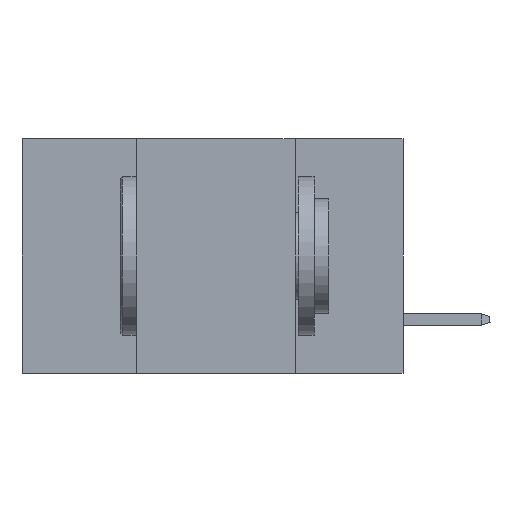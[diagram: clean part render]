
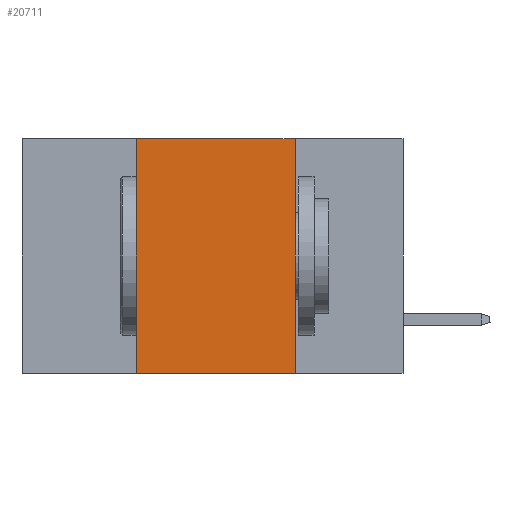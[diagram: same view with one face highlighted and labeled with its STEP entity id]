
A CAD part, left-side view. The second image highlights one B-rep face of the part: STEP entity #20711.
In plain terms, the highlighted planar face has unit normal (-1, 0, 0).
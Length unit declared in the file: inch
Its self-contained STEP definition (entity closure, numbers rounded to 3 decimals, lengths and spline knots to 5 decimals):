
#436 = EDGE_LOOP ( 'NONE', ( #23917, #10167, #9703, #27167 ) ) ;
#1954 = DIRECTION ( 'NONE',  ( 1., 0., 0. ) ) ;
#2016 = VECTOR ( 'NONE', #8291, 39.37008 ) ;
#4100 = VERTEX_POINT ( 'NONE', #9252 ) ;
#5850 = EDGE_CURVE ( 'NONE', #25699, #18921, #11287, .T. ) ;
#6035 = CARTESIAN_POINT ( 'NONE',  ( 0., 0.42, 0. ) ) ;
#6901 = EDGE_CURVE ( 'NONE', #18921, #4100, #20561, .T. ) ;
#7344 = DIRECTION ( 'NONE',  ( 0., -1., 0. ) ) ;
#7386 = DIRECTION ( 'NONE',  ( 0., -1., 0. ) ) ;
#8291 = DIRECTION ( 'NONE',  ( 0., 0., -1. ) ) ;
#9195 = CARTESIAN_POINT ( 'NONE',  ( 0., 0.6, -0.37 ) ) ;
#9252 = CARTESIAN_POINT ( 'NONE',  ( 0., 0.17, 0. ) ) ;
#9703 = ORIENTED_EDGE ( 'NONE', *, *, #5850, .F. ) ;
#9751 = VERTEX_POINT ( 'NONE', #16095 ) ;
#9924 = EDGE_CURVE ( 'NONE', #4100, #9751, #20961, .T. ) ;
#10167 = ORIENTED_EDGE ( 'NONE', *, *, #6901, .F. ) ;
#11287 = LINE ( 'NONE', #17707, #13833 ) ;
#11636 = CARTESIAN_POINT ( 'NONE',  ( 0., 0.6, 0. ) ) ;
#13833 = VECTOR ( 'NONE', #26372, 39.37008 ) ;
#14883 = VECTOR ( 'NONE', #7386, 39.37008 ) ;
#15274 = FACE_OUTER_BOUND ( 'NONE', #436, .T. ) ;
#16095 = CARTESIAN_POINT ( 'NONE',  ( 0., 0.17, -0.37 ) ) ;
#17707 = CARTESIAN_POINT ( 'NONE',  ( 0., 0.42, 0. ) ) ;
#17901 = CARTESIAN_POINT ( 'NONE',  ( 0., 0.42, -0.37 ) ) ;
#18889 = CARTESIAN_POINT ( 'NONE',  ( 0., 0.17, 0. ) ) ;
#18921 = VERTEX_POINT ( 'NONE', #6035 ) ;
#18944 = DIRECTION ( 'NONE',  ( 0., 0., -1. ) ) ;
#20561 = LINE ( 'NONE', #11636, #25492 ) ;
#20711 = ADVANCED_FACE ( 'NONE', ( #15274 ), #23803, .F. ) ;
#20961 = LINE ( 'NONE', #18889, #2016 ) ;
#21018 = CARTESIAN_POINT ( 'NONE',  ( 0., 0.6, 0. ) ) ;
#23803 = PLANE ( 'NONE',  #23933 ) ;
#23917 = ORIENTED_EDGE ( 'NONE', *, *, #9924, .F. ) ;
#23933 = AXIS2_PLACEMENT_3D ( 'NONE', #21018, #1954, #18944 ) ;
#24711 = EDGE_CURVE ( 'NONE', #25699, #9751, #26487, .T. ) ;
#25492 = VECTOR ( 'NONE', #7344, 39.37008 ) ;
#25699 = VERTEX_POINT ( 'NONE', #17901 ) ;
#26372 = DIRECTION ( 'NONE',  ( 0., 0., 1. ) ) ;
#26487 = LINE ( 'NONE', #9195, #14883 ) ;
#27167 = ORIENTED_EDGE ( 'NONE', *, *, #24711, .T. ) ;
